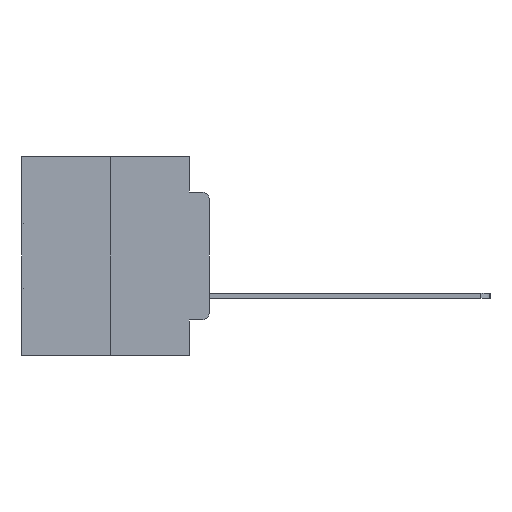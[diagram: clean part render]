
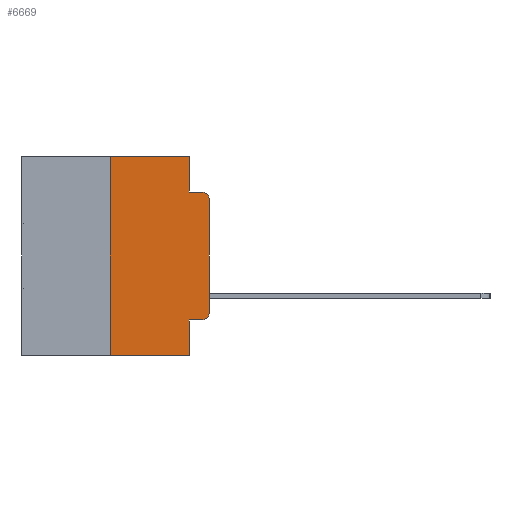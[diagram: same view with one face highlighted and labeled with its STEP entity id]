
A CAD part, left-side view. The second image highlights one B-rep face of the part: STEP entity #6669.
In plain terms, the highlighted planar face has unit normal (-1, 0, 0).
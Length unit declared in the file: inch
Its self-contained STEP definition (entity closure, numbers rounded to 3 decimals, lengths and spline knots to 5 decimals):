
#95 = CARTESIAN_POINT ( 'NONE',  ( 0., 0.051, 0. ) ) ;
#593 = EDGE_CURVE ( 'NONE', #19806, #19055, #19369, .T. ) ;
#672 = VECTOR ( 'NONE', #16919, 39.37008 ) ;
#723 = ORIENTED_EDGE ( 'NONE', *, *, #2064, .F. ) ;
#1381 = DIRECTION ( 'NONE',  ( 0., -1., 0. ) ) ;
#1774 = LINE ( 'NONE', #23002, #28158 ) ;
#1991 = LINE ( 'NONE', #17741, #13877 ) ;
#2064 = EDGE_CURVE ( 'NONE', #4021, #14439, #26619, .T. ) ;
#2216 = CARTESIAN_POINT ( 'NONE',  ( 0., 0.051, -0.0885 ) ) ;
#2321 = DIRECTION ( 'NONE',  ( 0., -1., 0. ) ) ;
#3763 = CARTESIAN_POINT ( 'NONE',  ( 0., 0.02, -0.1085 ) ) ;
#4021 = VERTEX_POINT ( 'NONE', #16534 ) ;
#4945 = ORIENTED_EDGE ( 'NONE', *, *, #26217, .T. ) ;
#4996 = EDGE_LOOP ( 'NONE', ( #27840, #4945, #7385, #19984, #723, #11960, #27693, #8340, #15179, #27798 ) ) ;
#6013 = DIRECTION ( 'NONE',  ( 0., 0., -1. ) ) ;
#6198 = CARTESIAN_POINT ( 'NONE',  ( 0., 0.473, 0. ) ) ;
#6266 = LINE ( 'NONE', #24917, #17416 ) ;
#6594 = DIRECTION ( 'NONE',  ( 0., 0., -1. ) ) ;
#6669 = ADVANCED_FACE ( 'NONE', ( #28129 ), #11486, .F. ) ;
#6684 = EDGE_CURVE ( 'NONE', #13479, #19055, #17443, .T. ) ;
#7118 = EDGE_CURVE ( 'NONE', #19806, #4021, #6266, .T. ) ;
#7385 = ORIENTED_EDGE ( 'NONE', *, *, #12913, .F. ) ;
#8340 = ORIENTED_EDGE ( 'NONE', *, *, #6684, .F. ) ;
#8802 = CARTESIAN_POINT ( 'NONE',  ( 0., 0.051, -0.5 ) ) ;
#8909 = DIRECTION ( 'NONE',  ( 1., 0., 0. ) ) ;
#9267 = VECTOR ( 'NONE', #1381, 39.37008 ) ;
#10185 = VECTOR ( 'NONE', #16272, 39.37008 ) ;
#10293 = CIRCLE ( 'NONE', #24454, 0.02 ) ;
#10871 = LINE ( 'NONE', #18491, #10185 ) ;
#11235 = CARTESIAN_POINT ( 'NONE',  ( 0., 0.02, -0.3915 ) ) ;
#11486 = PLANE ( 'NONE',  #13353 ) ;
#11960 = ORIENTED_EDGE ( 'NONE', *, *, #7118, .F. ) ;
#12913 = EDGE_CURVE ( 'NONE', #18236, #27359, #1991, .T. ) ;
#13232 = CARTESIAN_POINT ( 'NONE',  ( 0., 0.051, 0. ) ) ;
#13323 = CARTESIAN_POINT ( 'NONE',  ( 0., 0., -0.1085 ) ) ;
#13353 = AXIS2_PLACEMENT_3D ( 'NONE', #6198, #8909, #26772 ) ;
#13479 = VERTEX_POINT ( 'NONE', #21697 ) ;
#13516 = VECTOR ( 'NONE', #2321, 39.37008 ) ;
#13868 = DIRECTION ( 'NONE',  ( 0., 0., -1. ) ) ;
#13877 = VECTOR ( 'NONE', #19922, 39.37008 ) ;
#13940 = LINE ( 'NONE', #13232, #25451 ) ;
#14439 = VERTEX_POINT ( 'NONE', #16852 ) ;
#14453 = CARTESIAN_POINT ( 'NONE',  ( 0., 0.02, -0.4115 ) ) ;
#15179 = ORIENTED_EDGE ( 'NONE', *, *, #27837, .T. ) ;
#15339 = VERTEX_POINT ( 'NONE', #28386 ) ;
#16272 = DIRECTION ( 'NONE',  ( 0., 0., 1. ) ) ;
#16519 = EDGE_CURVE ( 'NONE', #15339, #27542, #10871, .T. ) ;
#16534 = CARTESIAN_POINT ( 'NONE',  ( 0., 0.25, 0. ) ) ;
#16616 = DIRECTION ( 'NONE',  ( 0., -1., 0. ) ) ;
#16852 = CARTESIAN_POINT ( 'NONE',  ( 0., 0.051, 0. ) ) ;
#16919 = DIRECTION ( 'NONE',  ( 0., 0., -1. ) ) ;
#17416 = VECTOR ( 'NONE', #19711, 39.37008 ) ;
#17443 = LINE ( 'NONE', #95, #672 ) ;
#17741 = CARTESIAN_POINT ( 'NONE',  ( 0., 0.051, -0.0885 ) ) ;
#18236 = VERTEX_POINT ( 'NONE', #2216 ) ;
#18491 = CARTESIAN_POINT ( 'NONE',  ( 0., 0., 0. ) ) ;
#19055 = VERTEX_POINT ( 'NONE', #8802 ) ;
#19298 = DIRECTION ( 'NONE',  ( -1., 0., 0. ) ) ;
#19369 = LINE ( 'NONE', #26245, #13516 ) ;
#19711 = DIRECTION ( 'NONE',  ( 0., 0., 1. ) ) ;
#19806 = VERTEX_POINT ( 'NONE', #20320 ) ;
#19922 = DIRECTION ( 'NONE',  ( 0., -1., 0. ) ) ;
#19984 = ORIENTED_EDGE ( 'NONE', *, *, #21335, .F. ) ;
#20320 = CARTESIAN_POINT ( 'NONE',  ( 0., 0.25, -0.5 ) ) ;
#21335 = EDGE_CURVE ( 'NONE', #14439, #18236, #13940, .T. ) ;
#21450 = CARTESIAN_POINT ( 'NONE',  ( 0., 0.02, -0.0885 ) ) ;
#21697 = CARTESIAN_POINT ( 'NONE',  ( 0., 0.051, -0.4115 ) ) ;
#21768 = AXIS2_PLACEMENT_3D ( 'NONE', #11235, #26812, #13868 ) ;
#22942 = CIRCLE ( 'NONE', #21768, 0.02 ) ;
#23002 = CARTESIAN_POINT ( 'NONE',  ( 0., 0.051, -0.4115 ) ) ;
#23077 = VERTEX_POINT ( 'NONE', #14453 ) ;
#24454 = AXIS2_PLACEMENT_3D ( 'NONE', #3763, #19298, #6013 ) ;
#24917 = CARTESIAN_POINT ( 'NONE',  ( 0., 0.25, 0. ) ) ;
#25318 = EDGE_CURVE ( 'NONE', #23077, #15339, #22942, .T. ) ;
#25451 = VECTOR ( 'NONE', #6594, 39.37008 ) ;
#26217 = EDGE_CURVE ( 'NONE', #27542, #27359, #10293, .T. ) ;
#26245 = CARTESIAN_POINT ( 'NONE',  ( 0., 0.473, -0.5 ) ) ;
#26619 = LINE ( 'NONE', #27597, #9267 ) ;
#26772 = DIRECTION ( 'NONE',  ( 0., 0., -1. ) ) ;
#26812 = DIRECTION ( 'NONE',  ( -1., 0., 0. ) ) ;
#27359 = VERTEX_POINT ( 'NONE', #21450 ) ;
#27542 = VERTEX_POINT ( 'NONE', #13323 ) ;
#27597 = CARTESIAN_POINT ( 'NONE',  ( 0., 0.473, 0. ) ) ;
#27693 = ORIENTED_EDGE ( 'NONE', *, *, #593, .T. ) ;
#27798 = ORIENTED_EDGE ( 'NONE', *, *, #25318, .T. ) ;
#27837 = EDGE_CURVE ( 'NONE', #13479, #23077, #1774, .T. ) ;
#27840 = ORIENTED_EDGE ( 'NONE', *, *, #16519, .T. ) ;
#28129 = FACE_OUTER_BOUND ( 'NONE', #4996, .T. ) ;
#28158 = VECTOR ( 'NONE', #16616, 39.37008 ) ;
#28386 = CARTESIAN_POINT ( 'NONE',  ( 0., 0., -0.3915 ) ) ;
